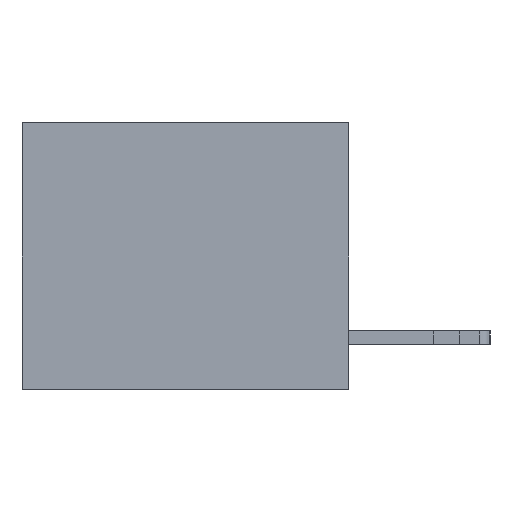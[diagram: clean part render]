
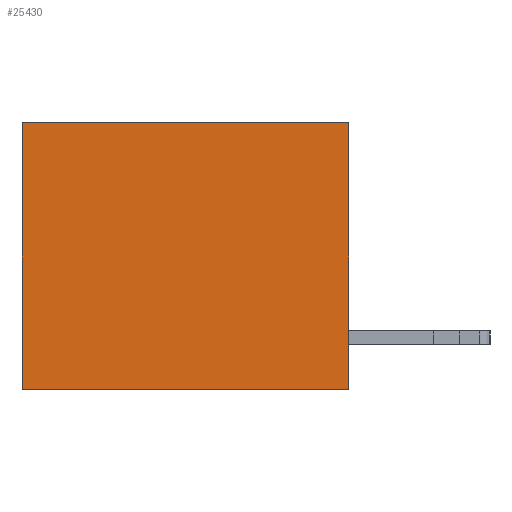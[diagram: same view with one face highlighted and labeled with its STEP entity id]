
A CAD part, left-side view. The second image highlights one B-rep face of the part: STEP entity #25430.
In plain terms, the highlighted planar face has unit normal (-1, 0, 0).
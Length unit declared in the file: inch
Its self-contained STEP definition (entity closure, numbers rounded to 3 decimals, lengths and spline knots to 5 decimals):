
#610 = ORIENTED_EDGE ( 'NONE', *, *, #2107, .F. ) ;
#995 = LINE ( 'NONE', #26962, #10197 ) ;
#2107 = EDGE_CURVE ( 'NONE', #5892, #20505, #23316, .T. ) ;
#2172 = CARTESIAN_POINT ( 'NONE',  ( 0.3165, 0., -0.49 ) ) ;
#2305 = VECTOR ( 'NONE', #25364, 39.37008 ) ;
#3237 = EDGE_CURVE ( 'NONE', #5892, #4290, #995, .T. ) ;
#4290 = VERTEX_POINT ( 'NONE', #9737 ) ;
#4454 = LINE ( 'NONE', #12177, #23173 ) ;
#4804 = CARTESIAN_POINT ( 'NONE',  ( 0.3165, 0., -0.49 ) ) ;
#5571 = EDGE_CURVE ( 'NONE', #4290, #13724, #8351, .T. ) ;
#5892 = VERTEX_POINT ( 'NONE', #22804 ) ;
#6572 = AXIS2_PLACEMENT_3D ( 'NONE', #4804, #25408, #11740 ) ;
#7190 = PLANE ( 'NONE',  #6572 ) ;
#7769 = CARTESIAN_POINT ( 'NONE',  ( 0.3165, 0.6, -0.49 ) ) ;
#8351 = LINE ( 'NONE', #9632, #2305 ) ;
#9207 = VECTOR ( 'NONE', #19874, 39.37008 ) ;
#9632 = CARTESIAN_POINT ( 'NONE',  ( 0.3165, 0.6, -0.49 ) ) ;
#9737 = CARTESIAN_POINT ( 'NONE',  ( 0.3165, 0.6, 0. ) ) ;
#10197 = VECTOR ( 'NONE', #19900, 39.37008 ) ;
#10617 = EDGE_CURVE ( 'NONE', #20505, #13724, #4454, .T. ) ;
#11740 = DIRECTION ( 'NONE',  ( 0., 0., -1. ) ) ;
#12137 = ORIENTED_EDGE ( 'NONE', *, *, #10617, .F. ) ;
#12177 = CARTESIAN_POINT ( 'NONE',  ( 0.3165, 0., -0.49 ) ) ;
#13724 = VERTEX_POINT ( 'NONE', #7769 ) ;
#18116 = CARTESIAN_POINT ( 'NONE',  ( 0.3165, 0., -0.49 ) ) ;
#19874 = DIRECTION ( 'NONE',  ( 0., 0., -1. ) ) ;
#19900 = DIRECTION ( 'NONE',  ( 0., 1., 0. ) ) ;
#20505 = VERTEX_POINT ( 'NONE', #18116 ) ;
#22804 = CARTESIAN_POINT ( 'NONE',  ( 0.3165, 0., 0. ) ) ;
#23173 = VECTOR ( 'NONE', #27865, 39.37008 ) ;
#23316 = LINE ( 'NONE', #2172, #9207 ) ;
#25360 = ORIENTED_EDGE ( 'NONE', *, *, #3237, .T. ) ;
#25364 = DIRECTION ( 'NONE',  ( 0., 0., -1. ) ) ;
#25408 = DIRECTION ( 'NONE',  ( 1., 0., 0. ) ) ;
#25430 = ADVANCED_FACE ( 'NONE', ( #26788 ), #7190, .F. ) ;
#25639 = ORIENTED_EDGE ( 'NONE', *, *, #5571, .T. ) ;
#26788 = FACE_OUTER_BOUND ( 'NONE', #26812, .T. ) ;
#26812 = EDGE_LOOP ( 'NONE', ( #25639, #12137, #610, #25360 ) ) ;
#26962 = CARTESIAN_POINT ( 'NONE',  ( 0.3165, 0., 0. ) ) ;
#27865 = DIRECTION ( 'NONE',  ( 0., 1., 0. ) ) ;
